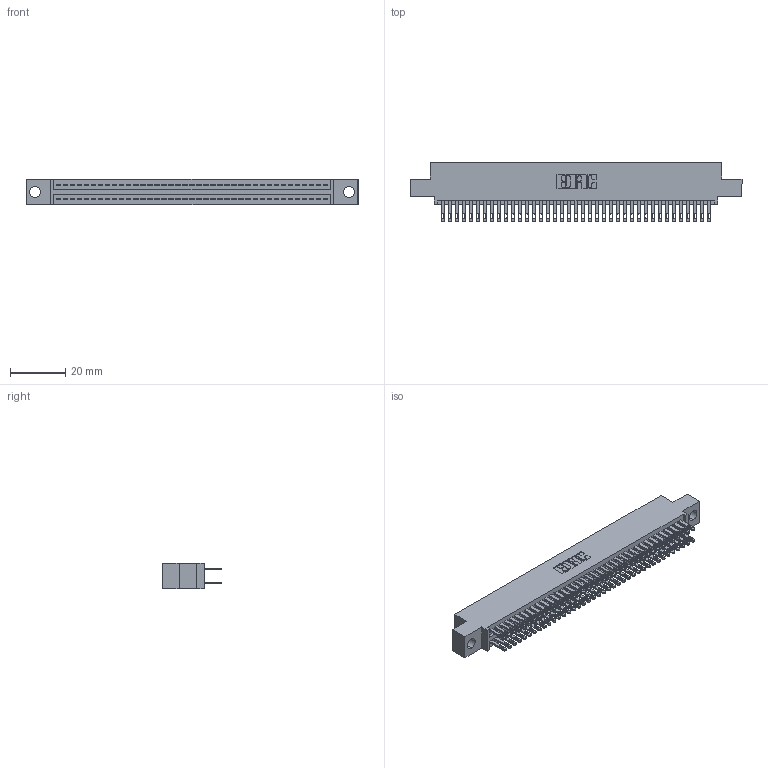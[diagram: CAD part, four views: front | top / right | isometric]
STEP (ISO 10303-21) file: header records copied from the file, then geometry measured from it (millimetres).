
FILE_DESCRIPTION (( 'STEP AP203' ), '1' );
FILE_NAME ('345-078-500-504.STEP', '2021-05-20T10:29:21', ( '' ), ( '' ), 'SwSTEP 2.0', 'SolidWorks 2020', '' );
FILE_SCHEMA (( 'CONFIG_CONTROL_DESIGN' ));
Length unit declared in the file: inch
Products named in the file (3): 345-078-500-504; 345-292-001_345-293-100; 345 Part_0.110 Offset - 0.156 Dia-TI
Assembly tree (79 placements, depth 2):
  345-078-500-504
    345 Part_0.110 Offset - 0.156 Dia-TI
    345-292-001_345-293-100  x78
Bounding box: 120.27 x 21.51 x 9.4 mm (x, y, z)
Volume: 11714.2 mm3; surface area: 17997.5 mm2
Topology: 79 solids, 79 shells, 3732 faces, 11387 edges, 7590 vertices
Faces by surface type: plane 2204, cylinder 1528
Entity records: 31485 total; most frequent: CARTESIAN_POINT 5286, ORIENTED_EDGE 5218, DIRECTION 4665, EDGE_CURVE 2609, VECTOR 2317, LINE 2317, VERTEX_POINT 1738, AXIS2_PLACEMENT_3D 1174
